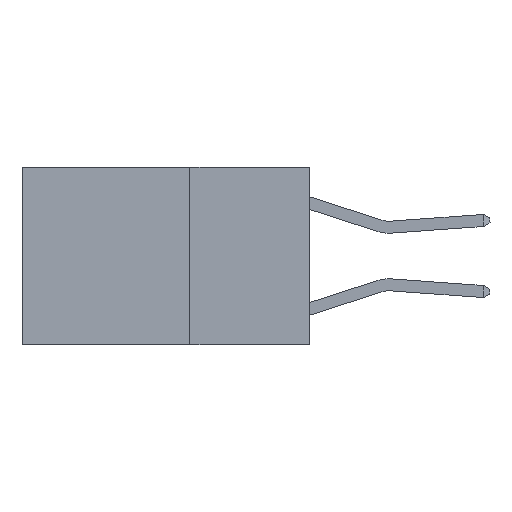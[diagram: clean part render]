
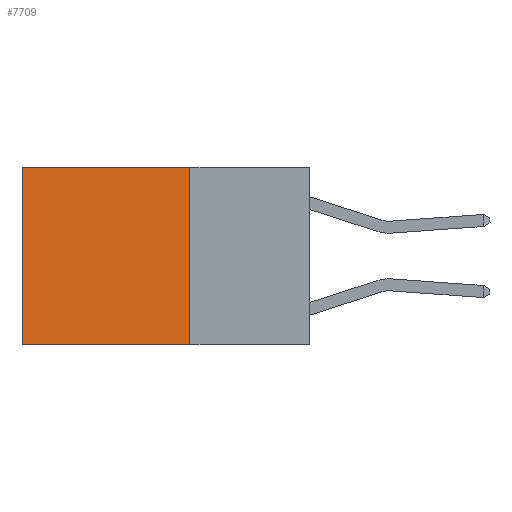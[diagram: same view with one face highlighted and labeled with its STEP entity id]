
A CAD part, left-side view. The second image highlights one B-rep face of the part: STEP entity #7709.
In plain terms, the highlighted planar face has unit normal (-1, 0, 0).
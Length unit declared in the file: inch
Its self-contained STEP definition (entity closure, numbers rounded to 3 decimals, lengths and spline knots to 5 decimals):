
#1 = EDGE_LOOP ( 'NONE', ( #5497, #5028, #6221, #8543 ) ) ;
#664 = LINE ( 'NONE', #4492, #4074 ) ;
#1220 = DIRECTION ( 'NONE',  ( 0., 1., 0. ) ) ;
#1420 = EDGE_CURVE ( 'NONE', #7304, #2789, #3491, .T. ) ;
#1800 = CARTESIAN_POINT ( 'NONE',  ( 0.2625, 0.25, 0. ) ) ;
#1996 = DIRECTION ( 'NONE',  ( 1., 0., 0. ) ) ;
#2215 = DIRECTION ( 'NONE',  ( 0., 1., 0. ) ) ;
#2789 = VERTEX_POINT ( 'NONE', #7422 ) ;
#2899 = CARTESIAN_POINT ( 'NONE',  ( 0.2625, 0.25, -0.37 ) ) ;
#2951 = LINE ( 'NONE', #2899, #6188 ) ;
#3490 = CARTESIAN_POINT ( 'NONE',  ( 0.2625, 0.6, -0.37 ) ) ;
#3491 = LINE ( 'NONE', #1800, #4988 ) ;
#4012 = PLANE ( 'NONE',  #4562 ) ;
#4029 = CARTESIAN_POINT ( 'NONE',  ( 0.2625, 0.25, 0. ) ) ;
#4074 = VECTOR ( 'NONE', #5148, 39.37008 ) ;
#4492 = CARTESIAN_POINT ( 'NONE',  ( 0.2625, 0.6, 0. ) ) ;
#4562 = AXIS2_PLACEMENT_3D ( 'NONE', #5967, #1996, #6585 ) ;
#4988 = VECTOR ( 'NONE', #1220, 39.37008 ) ;
#5028 = ORIENTED_EDGE ( 'NONE', *, *, #8659, .F. ) ;
#5148 = DIRECTION ( 'NONE',  ( 0., 0., -1. ) ) ;
#5394 = FACE_OUTER_BOUND ( 'NONE', #1, .T. ) ;
#5497 = ORIENTED_EDGE ( 'NONE', *, *, #8233, .T. ) ;
#5888 = EDGE_CURVE ( 'NONE', #7304, #6949, #7554, .T. ) ;
#5967 = CARTESIAN_POINT ( 'NONE',  ( 0.2625, 0.25, 0. ) ) ;
#6050 = VECTOR ( 'NONE', #7249, 39.37008 ) ;
#6188 = VECTOR ( 'NONE', #2215, 39.37008 ) ;
#6221 = ORIENTED_EDGE ( 'NONE', *, *, #5888, .F. ) ;
#6229 = CARTESIAN_POINT ( 'NONE',  ( 0.2625, 0.25, 0. ) ) ;
#6585 = DIRECTION ( 'NONE',  ( 0., 0., -1. ) ) ;
#6949 = VERTEX_POINT ( 'NONE', #7707 ) ;
#7249 = DIRECTION ( 'NONE',  ( 0., 0., -1. ) ) ;
#7304 = VERTEX_POINT ( 'NONE', #6229 ) ;
#7422 = CARTESIAN_POINT ( 'NONE',  ( 0.2625, 0.6, 0. ) ) ;
#7554 = LINE ( 'NONE', #4029, #6050 ) ;
#7707 = CARTESIAN_POINT ( 'NONE',  ( 0.2625, 0.25, -0.37 ) ) ;
#7709 = ADVANCED_FACE ( 'NONE', ( #5394 ), #4012, .F. ) ;
#8233 = EDGE_CURVE ( 'NONE', #2789, #8532, #664, .T. ) ;
#8532 = VERTEX_POINT ( 'NONE', #3490 ) ;
#8543 = ORIENTED_EDGE ( 'NONE', *, *, #1420, .T. ) ;
#8659 = EDGE_CURVE ( 'NONE', #6949, #8532, #2951, .T. ) ;
